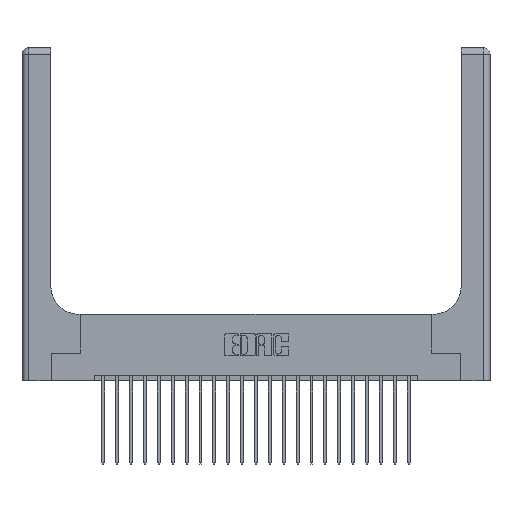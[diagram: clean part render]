
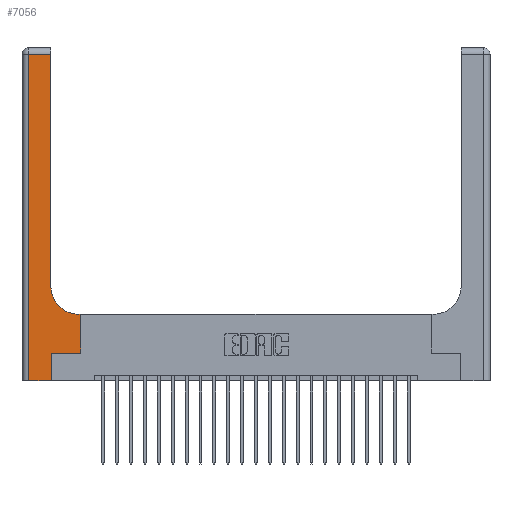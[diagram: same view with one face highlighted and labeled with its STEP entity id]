
A CAD part, top view. The second image highlights one B-rep face of the part: STEP entity #7056.
In plain terms, the highlighted planar face has unit normal (0, 0, 1).
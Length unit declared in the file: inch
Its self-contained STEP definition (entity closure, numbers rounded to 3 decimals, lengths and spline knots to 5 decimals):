
#736 = CARTESIAN_POINT ( 'NONE',  ( 0.26, 0.85, 0.37 ) ) ;
#1004 = EDGE_CURVE ( 'NONE', #6201, #15115, #19912, .T. ) ;
#1144 = EDGE_CURVE ( 'NONE', #11234, #6201, #5888, .T. ) ;
#1673 = VECTOR ( 'NONE', #20097, 39.37008 ) ;
#1791 = EDGE_CURVE ( 'NONE', #17073, #21684, #7763, .T. ) ;
#1996 = CARTESIAN_POINT ( 'NONE',  ( 0.06, 2.94, 0.37 ) ) ;
#2092 = CARTESIAN_POINT ( 'NONE',  ( 0., 2.94, 0.37 ) ) ;
#2421 = ORIENTED_EDGE ( 'NONE', *, *, #12095, .T. ) ;
#2461 = CARTESIAN_POINT ( 'NONE',  ( 0.06, 3., 0.37 ) ) ;
#2588 = DIRECTION ( 'NONE',  ( 1., 0., 0. ) ) ;
#2777 = EDGE_CURVE ( 'NONE', #15115, #5750, #20936, .T. ) ;
#2864 = DIRECTION ( 'NONE',  ( 0., 0., -1. ) ) ;
#3443 = ORIENTED_EDGE ( 'NONE', *, *, #1144, .T. ) ;
#3929 = EDGE_CURVE ( 'NONE', #5750, #17073, #11870, .T. ) ;
#4225 = ORIENTED_EDGE ( 'NONE', *, *, #1791, .T. ) ;
#4379 = CARTESIAN_POINT ( 'NONE',  ( 0.51, 0.85, 0.37 ) ) ;
#4541 = LINE ( 'NONE', #2092, #4816 ) ;
#4816 = VECTOR ( 'NONE', #17928, 39.37008 ) ;
#4993 = CARTESIAN_POINT ( 'NONE',  ( 0.528, 0.25, 0.37 ) ) ;
#5750 = VERTEX_POINT ( 'NONE', #19031 ) ;
#5888 = LINE ( 'NONE', #17112, #6180 ) ;
#5938 = CARTESIAN_POINT ( 'NONE',  ( 0.265, 0., 0.37 ) ) ;
#5947 = EDGE_CURVE ( 'NONE', #6167, #13322, #4541, .T. ) ;
#6167 = VERTEX_POINT ( 'NONE', #6521 ) ;
#6180 = VECTOR ( 'NONE', #10057, 39.37008 ) ;
#6201 = VERTEX_POINT ( 'NONE', #17884 ) ;
#6347 = CARTESIAN_POINT ( 'NONE',  ( 0., 3., 0.37 ) ) ;
#6521 = CARTESIAN_POINT ( 'NONE',  ( 0.26, 2.94, 0.37 ) ) ;
#6577 = DIRECTION ( 'NONE',  ( -1., 0., 0. ) ) ;
#6905 = LINE ( 'NONE', #2461, #1673 ) ;
#7056 = ADVANCED_FACE ( 'NONE', ( #7525 ), #10039, .F. ) ;
#7525 = FACE_OUTER_BOUND ( 'NONE', #17816, .T. ) ;
#7763 = LINE ( 'NONE', #15476, #18198 ) ;
#7975 = DIRECTION ( 'NONE',  ( 0., 1., 0. ) ) ;
#8705 = CARTESIAN_POINT ( 'NONE',  ( 0.528, 0.6, 0.37 ) ) ;
#9704 = DIRECTION ( 'NONE',  ( 0., 0., -1. ) ) ;
#10039 = PLANE ( 'NONE',  #13998 ) ;
#10057 = DIRECTION ( 'NONE',  ( 1., 0., 0. ) ) ;
#10932 = CARTESIAN_POINT ( 'NONE',  ( 0.265, 0.25, 0.37 ) ) ;
#11234 = VERTEX_POINT ( 'NONE', #20418 ) ;
#11479 = ORIENTED_EDGE ( 'NONE', *, *, #15577, .T. ) ;
#11870 = LINE ( 'NONE', #4993, #19675 ) ;
#11874 = CARTESIAN_POINT ( 'NONE',  ( 0.51, 0.6, 0.37 ) ) ;
#11876 = DIRECTION ( 'NONE',  ( -1., 0., 0. ) ) ;
#12095 = EDGE_CURVE ( 'NONE', #21684, #19212, #20728, .T. ) ;
#13322 = VERTEX_POINT ( 'NONE', #1996 ) ;
#13998 = AXIS2_PLACEMENT_3D ( 'NONE', #6347, #2864, #11876 ) ;
#15115 = VERTEX_POINT ( 'NONE', #10932 ) ;
#15197 = ORIENTED_EDGE ( 'NONE', *, *, #3929, .T. ) ;
#15222 = DIRECTION ( 'NONE',  ( 1., 0., 0. ) ) ;
#15476 = CARTESIAN_POINT ( 'NONE',  ( 0.26, 0.6, 0.37 ) ) ;
#15577 = EDGE_CURVE ( 'NONE', #19212, #6167, #21949, .T. ) ;
#16764 = CARTESIAN_POINT ( 'NONE',  ( 0.265, 0.25, 0.37 ) ) ;
#17073 = VERTEX_POINT ( 'NONE', #8705 ) ;
#17112 = CARTESIAN_POINT ( 'NONE',  ( 0., 0., 0.37 ) ) ;
#17137 = DIRECTION ( 'NONE',  ( 0., 1., 0. ) ) ;
#17816 = EDGE_LOOP ( 'NONE', ( #11479, #22549, #18828, #3443, #19930, #18963, #15197, #4225, #2421 ) ) ;
#17884 = CARTESIAN_POINT ( 'NONE',  ( 0.265, 0., 0.37 ) ) ;
#17928 = DIRECTION ( 'NONE',  ( -1., 0., 0. ) ) ;
#18198 = VECTOR ( 'NONE', #6577, 39.37008 ) ;
#18801 = VECTOR ( 'NONE', #19850, 39.37008 ) ;
#18828 = ORIENTED_EDGE ( 'NONE', *, *, #21100, .T. ) ;
#18963 = ORIENTED_EDGE ( 'NONE', *, *, #2777, .T. ) ;
#19031 = CARTESIAN_POINT ( 'NONE',  ( 0.528, 0.25, 0.37 ) ) ;
#19212 = VERTEX_POINT ( 'NONE', #736 ) ;
#19230 = AXIS2_PLACEMENT_3D ( 'NONE', #4379, #9704, #2588 ) ;
#19675 = VECTOR ( 'NONE', #17137, 39.37008 ) ;
#19850 = DIRECTION ( 'NONE',  ( 0., 1., 0. ) ) ;
#19912 = LINE ( 'NONE', #5938, #18801 ) ;
#19930 = ORIENTED_EDGE ( 'NONE', *, *, #1004, .T. ) ;
#20097 = DIRECTION ( 'NONE',  ( 0., -1., 0. ) ) ;
#20418 = CARTESIAN_POINT ( 'NONE',  ( 0.06, 0., 0.37 ) ) ;
#20503 = CARTESIAN_POINT ( 'NONE',  ( 0.26, 3., 0.37 ) ) ;
#20671 = VECTOR ( 'NONE', #15222, 39.37008 ) ;
#20728 = CIRCLE ( 'NONE', #19230, 0.25 ) ;
#20936 = LINE ( 'NONE', #16764, #20671 ) ;
#21100 = EDGE_CURVE ( 'NONE', #13322, #11234, #6905, .T. ) ;
#21657 = VECTOR ( 'NONE', #7975, 39.37008 ) ;
#21684 = VERTEX_POINT ( 'NONE', #11874 ) ;
#21949 = LINE ( 'NONE', #20503, #21657 ) ;
#22549 = ORIENTED_EDGE ( 'NONE', *, *, #5947, .T. ) ;
